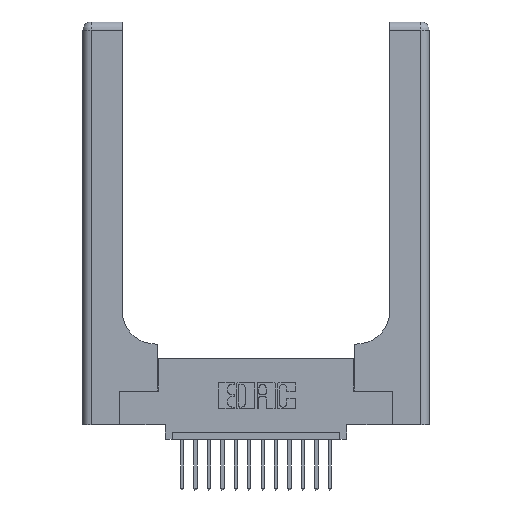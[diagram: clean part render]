
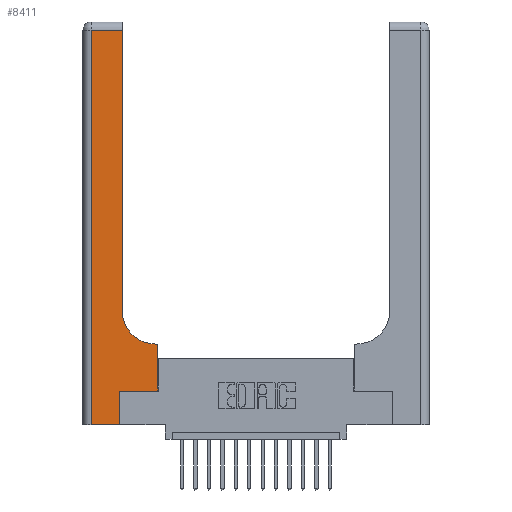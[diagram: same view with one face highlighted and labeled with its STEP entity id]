
A CAD part, top view. The second image highlights one B-rep face of the part: STEP entity #8411.
In plain terms, the highlighted planar face has unit normal (0, 0, 1).
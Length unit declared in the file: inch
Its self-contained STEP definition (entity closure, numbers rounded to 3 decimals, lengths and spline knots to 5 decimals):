
#59 = LINE ( 'NONE', #2060, #17406 ) ;
#397 = AXIS2_PLACEMENT_3D ( 'NONE', #14513, #14578, #1743 ) ;
#1293 = ORIENTED_EDGE ( 'NONE', *, *, #16993, .T. ) ;
#1553 = VECTOR ( 'NONE', #16170, 39.37008 ) ;
#1667 = VERTEX_POINT ( 'NONE', #17803 ) ;
#1692 = CARTESIAN_POINT ( 'NONE',  ( 0.5585, 0.6, 0.37 ) ) ;
#1743 = DIRECTION ( 'NONE',  ( 1., 0., 0. ) ) ;
#1957 = DIRECTION ( 'NONE',  ( 1., 0., 0. ) ) ;
#2060 = CARTESIAN_POINT ( 'NONE',  ( 0.269, 0., 0.37 ) ) ;
#2298 = EDGE_CURVE ( 'NONE', #13993, #1667, #13743, .T. ) ;
#2416 = CARTESIAN_POINT ( 'NONE',  ( 0.269, 0.25, 0.37 ) ) ;
#2758 = CARTESIAN_POINT ( 'NONE',  ( 0.269, 0.25, 0.37 ) ) ;
#3058 = EDGE_CURVE ( 'NONE', #10845, #12701, #15418, .T. ) ;
#3160 = EDGE_CURVE ( 'NONE', #3220, #11431, #7447, .T. ) ;
#3220 = VERTEX_POINT ( 'NONE', #10695 ) ;
#3686 = VERTEX_POINT ( 'NONE', #15199 ) ;
#3978 = EDGE_CURVE ( 'NONE', #8429, #13993, #10291, .T. ) ;
#4146 = VECTOR ( 'NONE', #13380, 39.37008 ) ;
#4258 = DIRECTION ( 'NONE',  ( 1., 0., 0. ) ) ;
#4789 = CARTESIAN_POINT ( 'NONE',  ( 0.269, 0., 0.37 ) ) ;
#4846 = VERTEX_POINT ( 'NONE', #2416 ) ;
#5341 = LINE ( 'NONE', #7639, #1553 ) ;
#5592 = VECTOR ( 'NONE', #17591, 39.37008 ) ;
#5952 = CARTESIAN_POINT ( 'NONE',  ( 0.2915, 2.94, 0.37 ) ) ;
#6268 = ORIENTED_EDGE ( 'NONE', *, *, #3058, .T. ) ;
#6446 = EDGE_CURVE ( 'NONE', #3686, #8429, #17766, .T. ) ;
#6527 = DIRECTION ( 'NONE',  ( 0., 0., -1. ) ) ;
#7447 = LINE ( 'NONE', #17067, #9864 ) ;
#7612 = DIRECTION ( 'NONE',  ( -1., 0., 0. ) ) ;
#7637 = CARTESIAN_POINT ( 'NONE',  ( 0.2915, 0.6, 0.37 ) ) ;
#7639 = CARTESIAN_POINT ( 'NONE',  ( 0.2915, 3., 0.37 ) ) ;
#8299 = EDGE_LOOP ( 'NONE', ( #17720, #6268, #17573, #13040, #1293, #12107, #17924, #18162, #15353 ) ) ;
#8411 = ADVANCED_FACE ( 'NONE', ( #9474 ), #12143, .F. ) ;
#8429 = VERTEX_POINT ( 'NONE', #1692 ) ;
#9474 = FACE_OUTER_BOUND ( 'NONE', #8299, .T. ) ;
#9864 = VECTOR ( 'NONE', #1957, 39.37008 ) ;
#10199 = AXIS2_PLACEMENT_3D ( 'NONE', #10841, #6527, #17845 ) ;
#10214 = CARTESIAN_POINT ( 'NONE',  ( 0.5415, 0.6, 0.37 ) ) ;
#10291 = LINE ( 'NONE', #7637, #4146 ) ;
#10695 = CARTESIAN_POINT ( 'NONE',  ( 0.06, 0., 0.37 ) ) ;
#10841 = CARTESIAN_POINT ( 'NONE',  ( 0., 3., 0.37 ) ) ;
#10845 = VERTEX_POINT ( 'NONE', #5952 ) ;
#11431 = VERTEX_POINT ( 'NONE', #4789 ) ;
#12107 = ORIENTED_EDGE ( 'NONE', *, *, #14966, .T. ) ;
#12143 = PLANE ( 'NONE',  #10199 ) ;
#12701 = VERTEX_POINT ( 'NONE', #15148 ) ;
#13040 = ORIENTED_EDGE ( 'NONE', *, *, #3160, .T. ) ;
#13307 = EDGE_CURVE ( 'NONE', #1667, #10845, #5341, .T. ) ;
#13380 = DIRECTION ( 'NONE',  ( -1., 0., 0. ) ) ;
#13506 = CARTESIAN_POINT ( 'NONE',  ( 0.5585, 0.25, 0.37 ) ) ;
#13743 = CIRCLE ( 'NONE', #397, 0.25 ) ;
#13879 = VECTOR ( 'NONE', #7612, 39.37008 ) ;
#13915 = VECTOR ( 'NONE', #4258, 39.37008 ) ;
#13993 = VERTEX_POINT ( 'NONE', #10214 ) ;
#14513 = CARTESIAN_POINT ( 'NONE',  ( 0.5415, 0.85, 0.37 ) ) ;
#14578 = DIRECTION ( 'NONE',  ( 0., 0., -1. ) ) ;
#14966 = EDGE_CURVE ( 'NONE', #4846, #3686, #17909, .T. ) ;
#15148 = CARTESIAN_POINT ( 'NONE',  ( 0.06, 2.94, 0.37 ) ) ;
#15199 = CARTESIAN_POINT ( 'NONE',  ( 0.5585, 0.25, 0.37 ) ) ;
#15353 = ORIENTED_EDGE ( 'NONE', *, *, #2298, .T. ) ;
#15364 = DIRECTION ( 'NONE',  ( 0., -1., 0. ) ) ;
#15418 = LINE ( 'NONE', #16088, #13879 ) ;
#16088 = CARTESIAN_POINT ( 'NONE',  ( 0., 2.94, 0.37 ) ) ;
#16170 = DIRECTION ( 'NONE',  ( 0., 1., 0. ) ) ;
#16356 = DIRECTION ( 'NONE',  ( 0., 1., 0. ) ) ;
#16501 = VECTOR ( 'NONE', #15364, 39.37008 ) ;
#16993 = EDGE_CURVE ( 'NONE', #11431, #4846, #59, .T. ) ;
#17067 = CARTESIAN_POINT ( 'NONE',  ( 0., 0., 0.37 ) ) ;
#17235 = EDGE_CURVE ( 'NONE', #12701, #3220, #18041, .T. ) ;
#17406 = VECTOR ( 'NONE', #16356, 39.37008 ) ;
#17573 = ORIENTED_EDGE ( 'NONE', *, *, #17235, .T. ) ;
#17591 = DIRECTION ( 'NONE',  ( 0., 1., 0. ) ) ;
#17720 = ORIENTED_EDGE ( 'NONE', *, *, #13307, .T. ) ;
#17766 = LINE ( 'NONE', #13506, #5592 ) ;
#17803 = CARTESIAN_POINT ( 'NONE',  ( 0.2915, 0.85, 0.37 ) ) ;
#17845 = DIRECTION ( 'NONE',  ( -1., 0., 0. ) ) ;
#17909 = LINE ( 'NONE', #2758, #13915 ) ;
#17924 = ORIENTED_EDGE ( 'NONE', *, *, #6446, .T. ) ;
#18037 = CARTESIAN_POINT ( 'NONE',  ( 0.06, 3., 0.37 ) ) ;
#18041 = LINE ( 'NONE', #18037, #16501 ) ;
#18162 = ORIENTED_EDGE ( 'NONE', *, *, #3978, .T. ) ;
